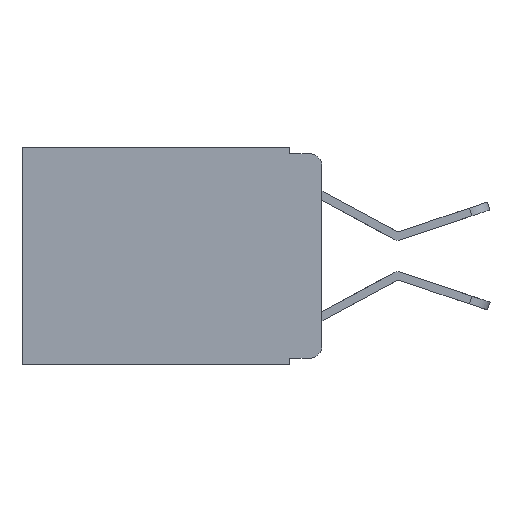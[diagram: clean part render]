
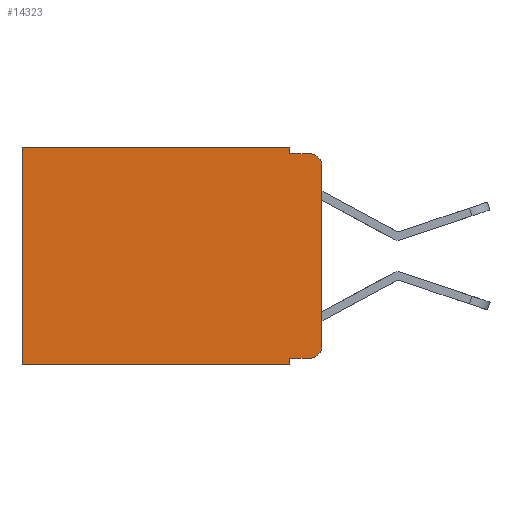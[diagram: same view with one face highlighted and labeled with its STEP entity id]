
A CAD part, left-side view. The second image highlights one B-rep face of the part: STEP entity #14323.
In plain terms, the highlighted planar face has unit normal (-1, 0, 0).
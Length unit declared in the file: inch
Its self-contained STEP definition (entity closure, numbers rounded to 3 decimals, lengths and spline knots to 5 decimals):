
#280 = LINE ( 'NONE', #16035, #11128 ) ;
#412 = DIRECTION ( 'NONE',  ( 0., -1., 0. ) ) ;
#441 = VECTOR ( 'NONE', #4857, 39.37008 ) ;
#502 = DIRECTION ( 'NONE',  ( -1., 0., 0. ) ) ;
#739 = VERTEX_POINT ( 'NONE', #9508 ) ;
#945 = VERTEX_POINT ( 'NONE', #3599 ) ;
#1380 = EDGE_CURVE ( 'NONE', #9655, #945, #15069, .T. ) ;
#1619 = CARTESIAN_POINT ( 'NONE',  ( 0.298, 0.02, -0.03 ) ) ;
#1620 = CARTESIAN_POINT ( 'NONE',  ( 0.298, 0.051, -0.01 ) ) ;
#1808 = VERTEX_POINT ( 'NONE', #9022 ) ;
#1891 = CARTESIAN_POINT ( 'NONE',  ( 0.298, 0.051, 0. ) ) ;
#1960 = CARTESIAN_POINT ( 'NONE',  ( 0.298, 0.051, 0. ) ) ;
#1996 = CARTESIAN_POINT ( 'NONE',  ( 0.298, 0.02, -0.333 ) ) ;
#2063 = DIRECTION ( 'NONE',  ( 0., 0., -1. ) ) ;
#2377 = CARTESIAN_POINT ( 'NONE',  ( 0.298, 0.051, -0.333 ) ) ;
#2717 = EDGE_CURVE ( 'NONE', #739, #8555, #13097, .T. ) ;
#2807 = DIRECTION ( 'NONE',  ( 0., 0., -1. ) ) ;
#2916 = DIRECTION ( 'NONE',  ( 0., 0., -1. ) ) ;
#3188 = LINE ( 'NONE', #1891, #11033 ) ;
#3338 = LINE ( 'NONE', #4688, #441 ) ;
#3382 = VERTEX_POINT ( 'NONE', #5069 ) ;
#3599 = CARTESIAN_POINT ( 'NONE',  ( 0.298, 0., -0.313 ) ) ;
#3689 = AXIS2_PLACEMENT_3D ( 'NONE', #1619, #502, #14808 ) ;
#3747 = CARTESIAN_POINT ( 'NONE',  ( 0.298, 0.473, 0. ) ) ;
#3749 = DIRECTION ( 'NONE',  ( 0., 0., -1. ) ) ;
#3774 = ORIENTED_EDGE ( 'NONE', *, *, #5586, .T. ) ;
#4075 = PLANE ( 'NONE',  #13550 ) ;
#4208 = ORIENTED_EDGE ( 'NONE', *, *, #16928, .T. ) ;
#4299 = DIRECTION ( 'NONE',  ( 0., 1., 0. ) ) ;
#4537 = VECTOR ( 'NONE', #412, 39.37008 ) ;
#4688 = CARTESIAN_POINT ( 'NONE',  ( 0.298, 0., -0.343 ) ) ;
#4857 = DIRECTION ( 'NONE',  ( 0., 1., 0. ) ) ;
#5047 = ORIENTED_EDGE ( 'NONE', *, *, #2717, .F. ) ;
#5069 = CARTESIAN_POINT ( 'NONE',  ( 0.298, 0.051, -0.343 ) ) ;
#5176 = FACE_OUTER_BOUND ( 'NONE', #5224, .T. ) ;
#5224 = EDGE_LOOP ( 'NONE', ( #8999, #3774, #5047, #10570, #16588, #4208, #15085, #6892, #13018, #8846 ) ) ;
#5586 = EDGE_CURVE ( 'NONE', #13519, #8555, #11071, .T. ) ;
#5587 = EDGE_CURVE ( 'NONE', #15540, #3382, #12227, .T. ) ;
#5708 = EDGE_CURVE ( 'NONE', #15540, #9655, #9754, .T. ) ;
#5785 = EDGE_CURVE ( 'NONE', #3382, #1808, #3338, .T. ) ;
#6306 = DIRECTION ( 'NONE',  ( -1., 0., 0. ) ) ;
#6669 = CARTESIAN_POINT ( 'NONE',  ( 0.298, 0.051, 0. ) ) ;
#6892 = ORIENTED_EDGE ( 'NONE', *, *, #5587, .F. ) ;
#8322 = EDGE_CURVE ( 'NONE', #13519, #945, #12003, .T. ) ;
#8555 = VERTEX_POINT ( 'NONE', #14053 ) ;
#8814 = CARTESIAN_POINT ( 'NONE',  ( 0.298, 0.473, 0. ) ) ;
#8846 = ORIENTED_EDGE ( 'NONE', *, *, #1380, .T. ) ;
#8999 = ORIENTED_EDGE ( 'NONE', *, *, #8322, .F. ) ;
#9022 = CARTESIAN_POINT ( 'NONE',  ( 0.298, 0.473, -0.343 ) ) ;
#9508 = CARTESIAN_POINT ( 'NONE',  ( 0.298, 0.051, -0.01 ) ) ;
#9655 = VERTEX_POINT ( 'NONE', #1996 ) ;
#9754 = LINE ( 'NONE', #14977, #4537 ) ;
#10008 = EDGE_CURVE ( 'NONE', #11565, #739, #3188, .T. ) ;
#10188 = DIRECTION ( 'NONE',  ( 0., 0., -1. ) ) ;
#10570 = ORIENTED_EDGE ( 'NONE', *, *, #10008, .F. ) ;
#10722 = VERTEX_POINT ( 'NONE', #3747 ) ;
#10810 = CARTESIAN_POINT ( 'NONE',  ( 0.298, 0., 0. ) ) ;
#10886 = VECTOR ( 'NONE', #11978, 39.37008 ) ;
#10975 = AXIS2_PLACEMENT_3D ( 'NONE', #11791, #6306, #3749 ) ;
#11033 = VECTOR ( 'NONE', #2063, 39.37008 ) ;
#11071 = CIRCLE ( 'NONE', #3689, 0.02 ) ;
#11128 = VECTOR ( 'NONE', #4299, 39.37008 ) ;
#11344 = VECTOR ( 'NONE', #12172, 39.37008 ) ;
#11565 = VERTEX_POINT ( 'NONE', #6669 ) ;
#11791 = CARTESIAN_POINT ( 'NONE',  ( 0.298, 0.02, -0.313 ) ) ;
#11978 = DIRECTION ( 'NONE',  ( 0., -1., 0. ) ) ;
#12003 = LINE ( 'NONE', #10810, #11344 ) ;
#12172 = DIRECTION ( 'NONE',  ( 0., 0., -1. ) ) ;
#12227 = LINE ( 'NONE', #1960, #13253 ) ;
#13018 = ORIENTED_EDGE ( 'NONE', *, *, #5708, .T. ) ;
#13097 = LINE ( 'NONE', #1620, #10886 ) ;
#13236 = DIRECTION ( 'NONE',  ( 1., 0., 0. ) ) ;
#13253 = VECTOR ( 'NONE', #2916, 39.37008 ) ;
#13519 = VERTEX_POINT ( 'NONE', #14873 ) ;
#13550 = AXIS2_PLACEMENT_3D ( 'NONE', #14525, #13236, #2807 ) ;
#13938 = VECTOR ( 'NONE', #10188, 39.37008 ) ;
#14053 = CARTESIAN_POINT ( 'NONE',  ( 0.298, 0.02, -0.01 ) ) ;
#14285 = LINE ( 'NONE', #8814, #13938 ) ;
#14323 = ADVANCED_FACE ( 'NONE', ( #5176 ), #4075, .F. ) ;
#14525 = CARTESIAN_POINT ( 'NONE',  ( 0.298, 0., 0. ) ) ;
#14808 = DIRECTION ( 'NONE',  ( 0., 0., -1. ) ) ;
#14866 = EDGE_CURVE ( 'NONE', #11565, #10722, #280, .T. ) ;
#14873 = CARTESIAN_POINT ( 'NONE',  ( 0.298, 0., -0.03 ) ) ;
#14977 = CARTESIAN_POINT ( 'NONE',  ( 0.298, 0.051, -0.333 ) ) ;
#15069 = CIRCLE ( 'NONE', #10975, 0.02 ) ;
#15085 = ORIENTED_EDGE ( 'NONE', *, *, #5785, .F. ) ;
#15540 = VERTEX_POINT ( 'NONE', #2377 ) ;
#16035 = CARTESIAN_POINT ( 'NONE',  ( 0.298, 0., 0. ) ) ;
#16588 = ORIENTED_EDGE ( 'NONE', *, *, #14866, .T. ) ;
#16928 = EDGE_CURVE ( 'NONE', #10722, #1808, #14285, .T. ) ;
